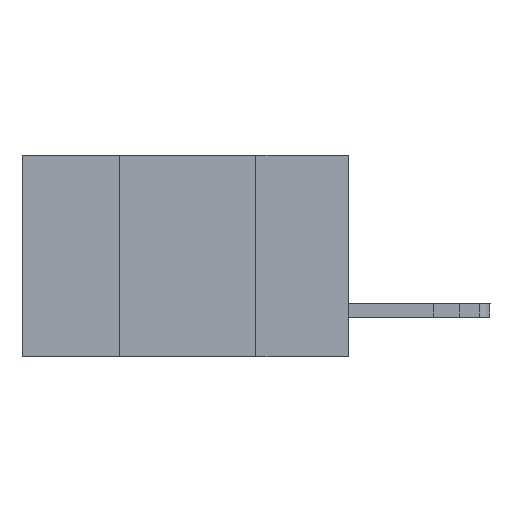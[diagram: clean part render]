
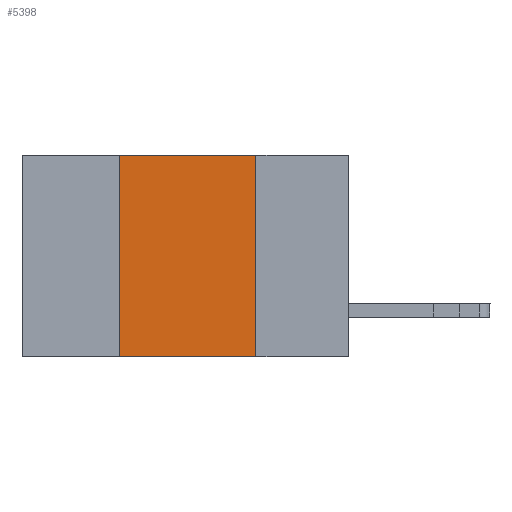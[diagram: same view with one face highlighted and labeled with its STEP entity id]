
A CAD part, left-side view. The second image highlights one B-rep face of the part: STEP entity #5398.
In plain terms, the highlighted planar face has unit normal (-1, 0, 0).
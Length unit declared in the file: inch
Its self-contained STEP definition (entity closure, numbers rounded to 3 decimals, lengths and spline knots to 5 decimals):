
#1015 = VERTEX_POINT ( 'NONE', #16015 ) ;
#2054 = DIRECTION ( 'NONE',  ( 1., 0., 0. ) ) ;
#2250 = LINE ( 'NONE', #7212, #8352 ) ;
#2415 = CARTESIAN_POINT ( 'NONE',  ( 0., 0.6, 0. ) ) ;
#2794 = VERTEX_POINT ( 'NONE', #5330 ) ;
#3120 = VECTOR ( 'NONE', #12367, 39.37008 ) ;
#3608 = CARTESIAN_POINT ( 'NONE',  ( 0., 0.6, 0. ) ) ;
#4103 = EDGE_CURVE ( 'NONE', #18416, #2794, #2250, .T. ) ;
#4583 = VECTOR ( 'NONE', #12359, 39.37008 ) ;
#5330 = CARTESIAN_POINT ( 'NONE',  ( 0., 0.17, -0.37 ) ) ;
#5398 = ADVANCED_FACE ( 'NONE', ( #11077 ), #11473, .F. ) ;
#7185 = EDGE_CURVE ( 'NONE', #1015, #2794, #9059, .T. ) ;
#7212 = CARTESIAN_POINT ( 'NONE',  ( 0., 0.6, -0.37 ) ) ;
#8352 = VECTOR ( 'NONE', #16202, 39.37008 ) ;
#9059 = LINE ( 'NONE', #12054, #3120 ) ;
#10077 = LINE ( 'NONE', #2415, #19779 ) ;
#10622 = CARTESIAN_POINT ( 'NONE',  ( 0., 0.42, 0. ) ) ;
#10713 = CARTESIAN_POINT ( 'NONE',  ( 0., 0.42, -0.37 ) ) ;
#11077 = FACE_OUTER_BOUND ( 'NONE', #19250, .T. ) ;
#11473 = PLANE ( 'NONE',  #13011 ) ;
#12054 = CARTESIAN_POINT ( 'NONE',  ( 0., 0.17, -0.37 ) ) ;
#12359 = DIRECTION ( 'NONE',  ( 0., 0., 1. ) ) ;
#12367 = DIRECTION ( 'NONE',  ( 0., 0., -1. ) ) ;
#13011 = AXIS2_PLACEMENT_3D ( 'NONE', #3608, #2054, #17368 ) ;
#13325 = CARTESIAN_POINT ( 'NONE',  ( 0., 0.42, -0.37 ) ) ;
#13360 = ORIENTED_EDGE ( 'NONE', *, *, #15164, .F. ) ;
#14250 = VERTEX_POINT ( 'NONE', #10622 ) ;
#14797 = EDGE_CURVE ( 'NONE', #18416, #14250, #15446, .T. ) ;
#14876 = ORIENTED_EDGE ( 'NONE', *, *, #7185, .F. ) ;
#15017 = DIRECTION ( 'NONE',  ( 0., -1., 0. ) ) ;
#15164 = EDGE_CURVE ( 'NONE', #14250, #1015, #10077, .T. ) ;
#15446 = LINE ( 'NONE', #10713, #4583 ) ;
#16015 = CARTESIAN_POINT ( 'NONE',  ( 0., 0.17, 0. ) ) ;
#16202 = DIRECTION ( 'NONE',  ( 0., -1., 0. ) ) ;
#17368 = DIRECTION ( 'NONE',  ( 0., 0., -1. ) ) ;
#18195 = ORIENTED_EDGE ( 'NONE', *, *, #4103, .T. ) ;
#18416 = VERTEX_POINT ( 'NONE', #13325 ) ;
#19250 = EDGE_LOOP ( 'NONE', ( #14876, #13360, #20059, #18195 ) ) ;
#19779 = VECTOR ( 'NONE', #15017, 39.37008 ) ;
#20059 = ORIENTED_EDGE ( 'NONE', *, *, #14797, .F. ) ;
